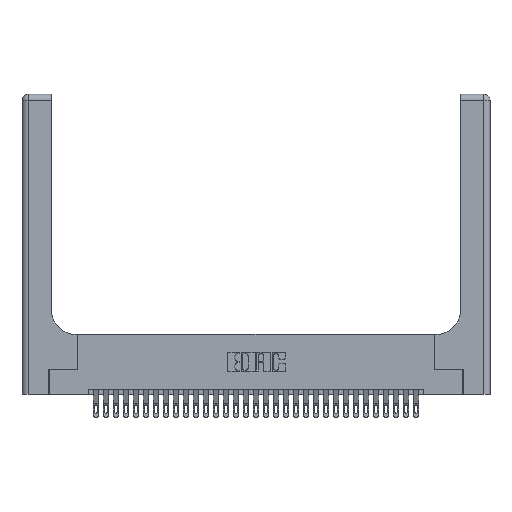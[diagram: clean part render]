
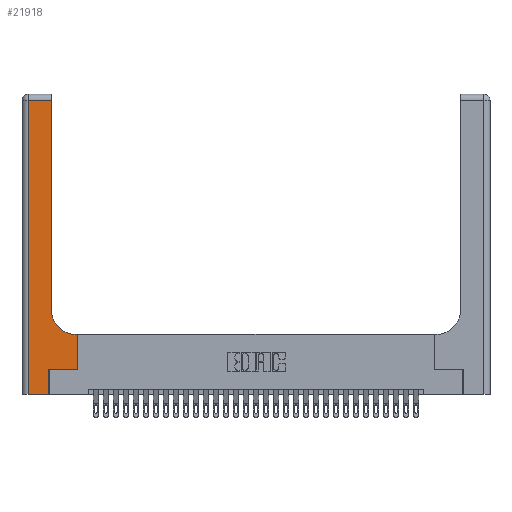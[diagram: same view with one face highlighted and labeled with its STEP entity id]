
A CAD part, top view. The second image highlights one B-rep face of the part: STEP entity #21918.
In plain terms, the highlighted planar face has unit normal (0, 0, 1).
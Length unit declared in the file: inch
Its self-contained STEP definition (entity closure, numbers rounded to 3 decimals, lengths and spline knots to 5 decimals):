
#195 = ORIENTED_EDGE ( 'NONE', *, *, #13907, .T. ) ;
#784 = LINE ( 'NONE', #11494, #1565 ) ;
#1405 = ORIENTED_EDGE ( 'NONE', *, *, #3373, .T. ) ;
#1565 = VECTOR ( 'NONE', #29341, 39.37008 ) ;
#1988 = DIRECTION ( 'NONE',  ( 0., 0., -1. ) ) ;
#2769 = DIRECTION ( 'NONE',  ( 0., -1., 0. ) ) ;
#3168 = VERTEX_POINT ( 'NONE', #20906 ) ;
#3373 = EDGE_CURVE ( 'NONE', #4261, #18895, #31883, .T. ) ;
#3833 = VECTOR ( 'NONE', #17619, 39.37008 ) ;
#4094 = CARTESIAN_POINT ( 'NONE',  ( 0.269, 0., 0.37 ) ) ;
#4261 = VERTEX_POINT ( 'NONE', #6301 ) ;
#4386 = PLANE ( 'NONE',  #10393 ) ;
#5776 = DIRECTION ( 'NONE',  ( 1., 0., 0. ) ) ;
#5955 = CARTESIAN_POINT ( 'NONE',  ( 0.2915, 0.6, 0.37 ) ) ;
#6301 = CARTESIAN_POINT ( 'NONE',  ( 0.5585, 0.6, 0.37 ) ) ;
#6615 = ORIENTED_EDGE ( 'NONE', *, *, #16963, .T. ) ;
#6941 = CARTESIAN_POINT ( 'NONE',  ( 0., 3., 0.37 ) ) ;
#7155 = DIRECTION ( 'NONE',  ( -1., 0., 0. ) ) ;
#7627 = LINE ( 'NONE', #17717, #13503 ) ;
#7736 = CARTESIAN_POINT ( 'NONE',  ( 0.5585, 0.25, 0.37 ) ) ;
#8198 = VERTEX_POINT ( 'NONE', #32344 ) ;
#8274 = CIRCLE ( 'NONE', #30059, 0.25 ) ;
#8455 = LINE ( 'NONE', #25880, #27718 ) ;
#8960 = VERTEX_POINT ( 'NONE', #25391 ) ;
#9041 = VECTOR ( 'NONE', #32244, 39.37008 ) ;
#10393 = AXIS2_PLACEMENT_3D ( 'NONE', #6941, #1988, #7155 ) ;
#10740 = ORIENTED_EDGE ( 'NONE', *, *, #22333, .T. ) ;
#11494 = CARTESIAN_POINT ( 'NONE',  ( 0.2915, 3., 0.37 ) ) ;
#11787 = DIRECTION ( 'NONE',  ( 0., 0., -1. ) ) ;
#13503 = VECTOR ( 'NONE', #2769, 39.37008 ) ;
#13907 = EDGE_CURVE ( 'NONE', #18895, #8198, #8274, .T. ) ;
#14018 = EDGE_CURVE ( 'NONE', #23267, #4261, #14816, .T. ) ;
#14288 = VECTOR ( 'NONE', #23977, 39.37008 ) ;
#14816 = LINE ( 'NONE', #7736, #3833 ) ;
#15729 = LINE ( 'NONE', #31620, #9041 ) ;
#15778 = ORIENTED_EDGE ( 'NONE', *, *, #14018, .T. ) ;
#15847 = CARTESIAN_POINT ( 'NONE',  ( 0.5585, 0.25, 0.37 ) ) ;
#16188 = CARTESIAN_POINT ( 'NONE',  ( 0.06, 0., 0.37 ) ) ;
#16548 = EDGE_CURVE ( 'NONE', #25493, #3168, #8455, .T. ) ;
#16963 = EDGE_CURVE ( 'NONE', #8960, #25493, #7627, .T. ) ;
#17156 = DIRECTION ( 'NONE',  ( 1., 0., 0. ) ) ;
#17533 = CARTESIAN_POINT ( 'NONE',  ( 0.269, 0.25, 0.37 ) ) ;
#17619 = DIRECTION ( 'NONE',  ( 0., 1., 0. ) ) ;
#17717 = CARTESIAN_POINT ( 'NONE',  ( 0.06, 3., 0.37 ) ) ;
#17801 = ORIENTED_EDGE ( 'NONE', *, *, #30110, .T. ) ;
#17841 = ORIENTED_EDGE ( 'NONE', *, *, #23837, .T. ) ;
#18895 = VERTEX_POINT ( 'NONE', #31644 ) ;
#19149 = VECTOR ( 'NONE', #17156, 39.37008 ) ;
#20203 = LINE ( 'NONE', #4094, #14288 ) ;
#20475 = FACE_OUTER_BOUND ( 'NONE', #28297, .T. ) ;
#20906 = CARTESIAN_POINT ( 'NONE',  ( 0.269, 0., 0.37 ) ) ;
#21493 = CARTESIAN_POINT ( 'NONE',  ( 0.5415, 0.85, 0.37 ) ) ;
#21887 = EDGE_CURVE ( 'NONE', #26710, #8960, #15729, .T. ) ;
#21918 = ADVANCED_FACE ( 'NONE', ( #20475 ), #4386, .F. ) ;
#22333 = EDGE_CURVE ( 'NONE', #8198, #26710, #784, .T. ) ;
#23267 = VERTEX_POINT ( 'NONE', #15847 ) ;
#23837 = EDGE_CURVE ( 'NONE', #28645, #23267, #24680, .T. ) ;
#23977 = DIRECTION ( 'NONE',  ( 0., 1., 0. ) ) ;
#24680 = LINE ( 'NONE', #24753, #19149 ) ;
#24753 = CARTESIAN_POINT ( 'NONE',  ( 0.269, 0.25, 0.37 ) ) ;
#25391 = CARTESIAN_POINT ( 'NONE',  ( 0.06, 2.94, 0.37 ) ) ;
#25493 = VERTEX_POINT ( 'NONE', #16188 ) ;
#25880 = CARTESIAN_POINT ( 'NONE',  ( 0., 0., 0.37 ) ) ;
#26058 = DIRECTION ( 'NONE',  ( -1., 0., 0. ) ) ;
#26710 = VERTEX_POINT ( 'NONE', #29441 ) ;
#27718 = VECTOR ( 'NONE', #5776, 39.37008 ) ;
#28297 = EDGE_LOOP ( 'NONE', ( #10740, #30801, #6615, #29849, #17801, #17841, #15778, #1405, #195 ) ) ;
#28645 = VERTEX_POINT ( 'NONE', #17533 ) ;
#29341 = DIRECTION ( 'NONE',  ( 0., 1., 0. ) ) ;
#29428 = DIRECTION ( 'NONE',  ( 1., 0., 0. ) ) ;
#29441 = CARTESIAN_POINT ( 'NONE',  ( 0.2915, 2.94, 0.37 ) ) ;
#29849 = ORIENTED_EDGE ( 'NONE', *, *, #16548, .T. ) ;
#30059 = AXIS2_PLACEMENT_3D ( 'NONE', #21493, #11787, #29428 ) ;
#30110 = EDGE_CURVE ( 'NONE', #3168, #28645, #20203, .T. ) ;
#30801 = ORIENTED_EDGE ( 'NONE', *, *, #21887, .T. ) ;
#31512 = VECTOR ( 'NONE', #26058, 39.37008 ) ;
#31620 = CARTESIAN_POINT ( 'NONE',  ( 0., 2.94, 0.37 ) ) ;
#31644 = CARTESIAN_POINT ( 'NONE',  ( 0.5415, 0.6, 0.37 ) ) ;
#31883 = LINE ( 'NONE', #5955, #31512 ) ;
#32244 = DIRECTION ( 'NONE',  ( -1., 0., 0. ) ) ;
#32344 = CARTESIAN_POINT ( 'NONE',  ( 0.2915, 0.85, 0.37 ) ) ;
